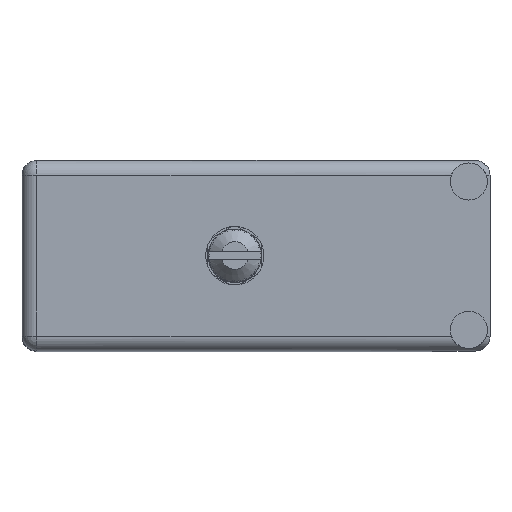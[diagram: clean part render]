
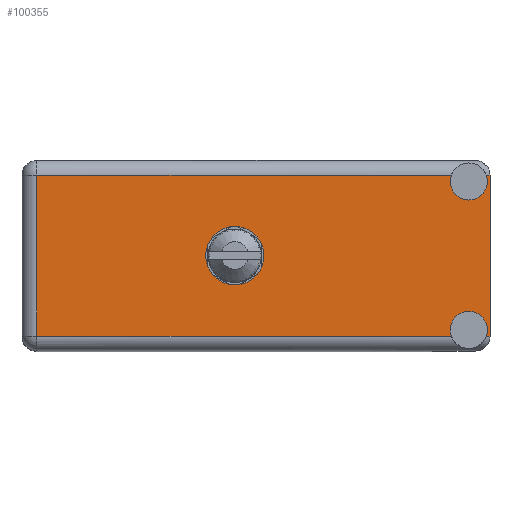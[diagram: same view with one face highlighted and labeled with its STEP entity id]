
A CAD part, top view. The second image highlights one B-rep face of the part: STEP entity #100355.
In plain terms, the highlighted face is planar.
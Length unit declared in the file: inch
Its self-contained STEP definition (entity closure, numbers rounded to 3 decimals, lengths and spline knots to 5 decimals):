
#367 = LINE ( 'NONE', #79721, #82672 ) ;
#5298 = ORIENTED_EDGE ( 'NONE', *, *, #102974, .F. ) ;
#5462 = DIRECTION ( 'NONE',  ( 0., 0., 1. ) ) ;
#5487 = CARTESIAN_POINT ( 'NONE',  ( 2.02562, 1.566, -0.07 ) ) ;
#6049 = DIRECTION ( 'NONE',  ( 0., 0., 1. ) ) ;
#8648 = CARTESIAN_POINT ( 'NONE',  ( 2.19038, 1.566, -0.07 ) ) ;
#9359 = ORIENTED_EDGE ( 'NONE', *, *, #75070, .T. ) ;
#10280 = LINE ( 'NONE', #110621, #69233 ) ;
#10771 = VERTEX_POINT ( 'NONE', #52670 ) ;
#10935 = AXIS2_PLACEMENT_3D ( 'NONE', #21966, #83260, #39551 ) ;
#13106 = FACE_OUTER_BOUND ( 'NONE', #113460, .T. ) ;
#14169 = DIRECTION ( 'NONE',  ( 0., 1., 0. ) ) ;
#16900 = LINE ( 'NONE', #37569, #42911 ) ;
#17651 = CIRCLE ( 'NONE', #10935, 0.0875 ) ;
#18790 = VERTEX_POINT ( 'NONE', #103604 ) ;
#20692 = PLANE ( 'NONE',  #31972 ) ;
#21925 = CARTESIAN_POINT ( 'NONE',  ( 2.208, 1.566, -0.07 ) ) ;
#21966 = CARTESIAN_POINT ( 'NONE',  ( 2.108, 1.566, -0.7995 ) ) ;
#23224 = EDGE_CURVE ( 'NONE', #18790, #64636, #17651, .T. ) ;
#26168 = LINE ( 'NONE', #44256, #109768 ) ;
#29424 = CARTESIAN_POINT ( 'NONE',  ( 2.208, 1.566, -0.829 ) ) ;
#30260 = DIRECTION ( 'NONE',  ( 0., 0., 1. ) ) ;
#30672 = CIRCLE ( 'NONE', #92196, 0.0875 ) ;
#30966 = EDGE_CURVE ( 'NONE', #37586, #106799, #41940, .T. ) ;
#31051 = CARTESIAN_POINT ( 'NONE',  ( 2.108, 1.566, -0.0995 ) ) ;
#31803 = DIRECTION ( 'NONE',  ( 0., 1., 0. ) ) ;
#31942 = CARTESIAN_POINT ( 'NONE',  ( 2.108, 1.566, -0.187 ) ) ;
#31972 = AXIS2_PLACEMENT_3D ( 'NONE', #82357, #82769, #30260 ) ;
#32193 = DIRECTION ( 'NONE',  ( 0., 0., 1. ) ) ;
#33323 = ORIENTED_EDGE ( 'NONE', *, *, #107621, .F. ) ;
#33450 = CARTESIAN_POINT ( 'NONE',  ( 2.19038, 1.566, -0.829 ) ) ;
#36231 = VERTEX_POINT ( 'NONE', #33450 ) ;
#37569 = CARTESIAN_POINT ( 'NONE',  ( 0., 1.566, -0.829 ) ) ;
#37586 = VERTEX_POINT ( 'NONE', #8648 ) ;
#39019 = CARTESIAN_POINT ( 'NONE',  ( 0.07, 1.566, -0.07 ) ) ;
#39515 = CARTESIAN_POINT ( 'NONE',  ( 2.208, 1.566, 0. ) ) ;
#39551 = DIRECTION ( 'NONE',  ( 0., 0., 1. ) ) ;
#39877 = DIRECTION ( 'NONE',  ( 0., 0., 1. ) ) ;
#40896 = EDGE_CURVE ( 'NONE', #72860, #10771, #110630, .T. ) ;
#41940 = CIRCLE ( 'NONE', #71962, 0.0875 ) ;
#42073 = EDGE_CURVE ( 'NONE', #37586, #108106, #10280, .T. ) ;
#42713 = ORIENTED_EDGE ( 'NONE', *, *, #40896, .F. ) ;
#42911 = VECTOR ( 'NONE', #55120, 39.37008 ) ;
#43779 = EDGE_CURVE ( 'NONE', #18790, #61107, #16900, .T. ) ;
#43829 = DIRECTION ( 'NONE',  ( 0., 0., 1. ) ) ;
#44256 = CARTESIAN_POINT ( 'NONE',  ( 0.07, 1.566, -0.899 ) ) ;
#48319 = LINE ( 'NONE', #39515, #79946 ) ;
#50479 = CARTESIAN_POINT ( 'NONE',  ( 1.004, 1.566, -0.4495 ) ) ;
#51143 = LINE ( 'NONE', #105066, #73030 ) ;
#52464 = CIRCLE ( 'NONE', #93014, 0.0875 ) ;
#52670 = CARTESIAN_POINT ( 'NONE',  ( 1.004, 1.566, -0.587 ) ) ;
#54363 = DIRECTION ( 'NONE',  ( 0., 0., 1. ) ) ;
#55120 = DIRECTION ( 'NONE',  ( -1., 0., 0. ) ) ;
#56887 = EDGE_CURVE ( 'NONE', #60012, #36231, #367, .T. ) ;
#57261 = DIRECTION ( 'NONE',  ( 1., 0., 0. ) ) ;
#58000 = DIRECTION ( 'NONE',  ( 0., 1., 0. ) ) ;
#60012 = VERTEX_POINT ( 'NONE', #29424 ) ;
#60057 = ORIENTED_EDGE ( 'NONE', *, *, #56887, .T. ) ;
#60886 = DIRECTION ( 'NONE',  ( 1., 0., 0. ) ) ;
#61107 = VERTEX_POINT ( 'NONE', #65352 ) ;
#61480 = CARTESIAN_POINT ( 'NONE',  ( 2.108, 1.566, -0.0995 ) ) ;
#62851 = DIRECTION ( 'NONE',  ( 0., 1., 0. ) ) ;
#64590 = AXIS2_PLACEMENT_3D ( 'NONE', #50479, #31803, #32193 ) ;
#64636 = VERTEX_POINT ( 'NONE', #111292 ) ;
#65352 = CARTESIAN_POINT ( 'NONE',  ( 0.07, 1.566, -0.829 ) ) ;
#65541 = EDGE_CURVE ( 'NONE', #10771, #72860, #73140, .T. ) ;
#69233 = VECTOR ( 'NONE', #57261, 39.37008 ) ;
#69329 = AXIS2_PLACEMENT_3D ( 'NONE', #110598, #58000, #5462 ) ;
#70151 = DIRECTION ( 'NONE',  ( -1., 0., 0. ) ) ;
#70305 = DIRECTION ( 'NONE',  ( 0., 1., 0. ) ) ;
#71962 = AXIS2_PLACEMENT_3D ( 'NONE', #31051, #14169, #6049 ) ;
#72860 = VERTEX_POINT ( 'NONE', #106198 ) ;
#73030 = VECTOR ( 'NONE', #60886, 39.37008 ) ;
#73140 = CIRCLE ( 'NONE', #64590, 0.1375 ) ;
#74869 = EDGE_CURVE ( 'NONE', #64636, #36231, #52464, .T. ) ;
#75070 = EDGE_CURVE ( 'NONE', #87979, #83426, #51143, .T. ) ;
#79721 = CARTESIAN_POINT ( 'NONE',  ( 0., 1.566, -0.829 ) ) ;
#79946 = VECTOR ( 'NONE', #39877, 39.37008 ) ;
#82357 = CARTESIAN_POINT ( 'NONE',  ( 0., 1.566, -0.899 ) ) ;
#82672 = VECTOR ( 'NONE', #70151, 39.37008 ) ;
#82769 = DIRECTION ( 'NONE',  ( 0., 1., 0. ) ) ;
#83260 = DIRECTION ( 'NONE',  ( 0., 1., 0. ) ) ;
#83317 = EDGE_CURVE ( 'NONE', #61107, #87979, #26168, .T. ) ;
#83426 = VERTEX_POINT ( 'NONE', #5487 ) ;
#85773 = ORIENTED_EDGE ( 'NONE', *, *, #43779, .T. ) ;
#87979 = VERTEX_POINT ( 'NONE', #39019 ) ;
#92196 = AXIS2_PLACEMENT_3D ( 'NONE', #61480, #70305, #43829 ) ;
#92226 = ORIENTED_EDGE ( 'NONE', *, *, #42073, .T. ) ;
#93014 = AXIS2_PLACEMENT_3D ( 'NONE', #98923, #62851, #54363 ) ;
#93593 = ORIENTED_EDGE ( 'NONE', *, *, #30966, .F. ) ;
#97149 = ORIENTED_EDGE ( 'NONE', *, *, #74869, .F. ) ;
#98923 = CARTESIAN_POINT ( 'NONE',  ( 2.108, 1.566, -0.7995 ) ) ;
#100355 = ADVANCED_FACE ( 'NONE', ( #106410, #13106 ), #20692, .T. ) ;
#101206 = EDGE_LOOP ( 'NONE', ( #42713, #111459 ) ) ;
#102974 = EDGE_CURVE ( 'NONE', #60012, #108106, #48319, .T. ) ;
#103604 = CARTESIAN_POINT ( 'NONE',  ( 2.02562, 1.566, -0.829 ) ) ;
#104606 = DIRECTION ( 'NONE',  ( 0., 0., 1. ) ) ;
#104646 = ORIENTED_EDGE ( 'NONE', *, *, #23224, .F. ) ;
#104841 = ORIENTED_EDGE ( 'NONE', *, *, #83317, .T. ) ;
#105066 = CARTESIAN_POINT ( 'NONE',  ( 2.208, 1.566, -0.07 ) ) ;
#106198 = CARTESIAN_POINT ( 'NONE',  ( 1.004, 1.566, -0.312 ) ) ;
#106410 = FACE_BOUND ( 'NONE', #101206, .T. ) ;
#106799 = VERTEX_POINT ( 'NONE', #31942 ) ;
#107621 = EDGE_CURVE ( 'NONE', #106799, #83426, #30672, .T. ) ;
#108106 = VERTEX_POINT ( 'NONE', #21925 ) ;
#109768 = VECTOR ( 'NONE', #104606, 39.37008 ) ;
#110598 = CARTESIAN_POINT ( 'NONE',  ( 1.004, 1.566, -0.4495 ) ) ;
#110621 = CARTESIAN_POINT ( 'NONE',  ( 2.208, 1.566, -0.07 ) ) ;
#110630 = CIRCLE ( 'NONE', #69329, 0.1375 ) ;
#111292 = CARTESIAN_POINT ( 'NONE',  ( 2.108, 1.566, -0.712 ) ) ;
#111459 = ORIENTED_EDGE ( 'NONE', *, *, #65541, .F. ) ;
#113460 = EDGE_LOOP ( 'NONE', ( #9359, #33323, #93593, #92226, #5298, #60057, #97149, #104646, #85773, #104841 ) ) ;
